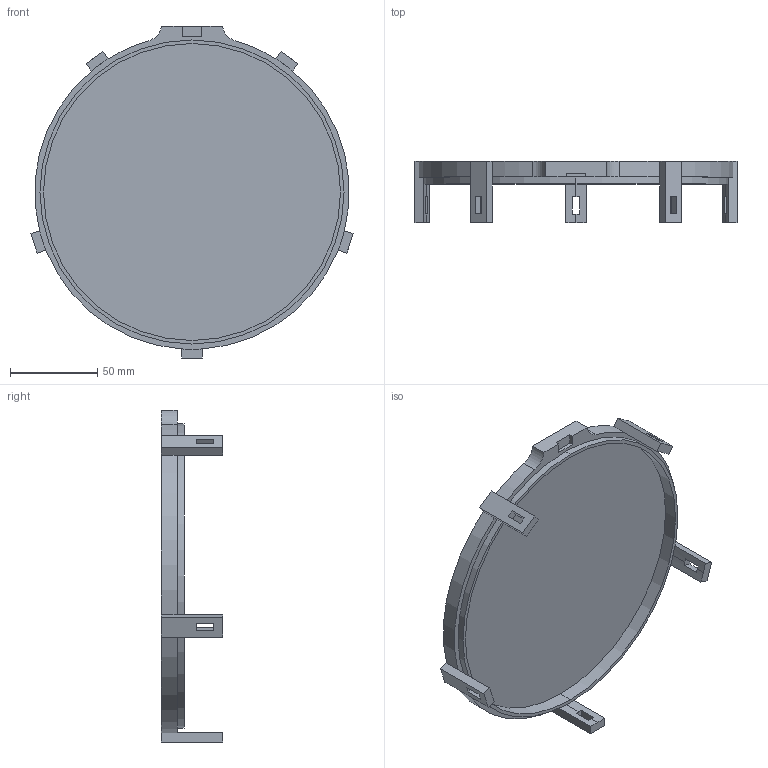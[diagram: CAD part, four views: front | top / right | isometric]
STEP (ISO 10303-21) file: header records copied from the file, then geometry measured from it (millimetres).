
FILE_DESCRIPTION (( 'STEP AP214' ), '1' );
FILE_NAME ('rear.STEP', '2013-12-22T02:48:42', ( '' ), ( '' ), 'SwSTEP 2.0', 'SolidWorks 2013', '' );
FILE_SCHEMA (( 'AUTOMOTIVE_DESIGN' ));
Length unit declared in the file: millimetre
Products named in the file (1): rear
Bounding box: 184.34 x 35 x 190 mm (x, y, z)
Volume: 153788.8 mm3; surface area: 68752.6 mm2
Topology: 1 solids, 1 shells, 71 faces, 206 edges, 134 vertices
Faces by surface type: plane 49, cylinder 22
Entity records: 2398 total; most frequent: DIRECTION 414, ORIENTED_EDGE 412, CARTESIAN_POINT 412, EDGE_CURVE 206, LINE 142, VECTOR 142, AXIS2_PLACEMENT_3D 136, VERTEX_POINT 134
